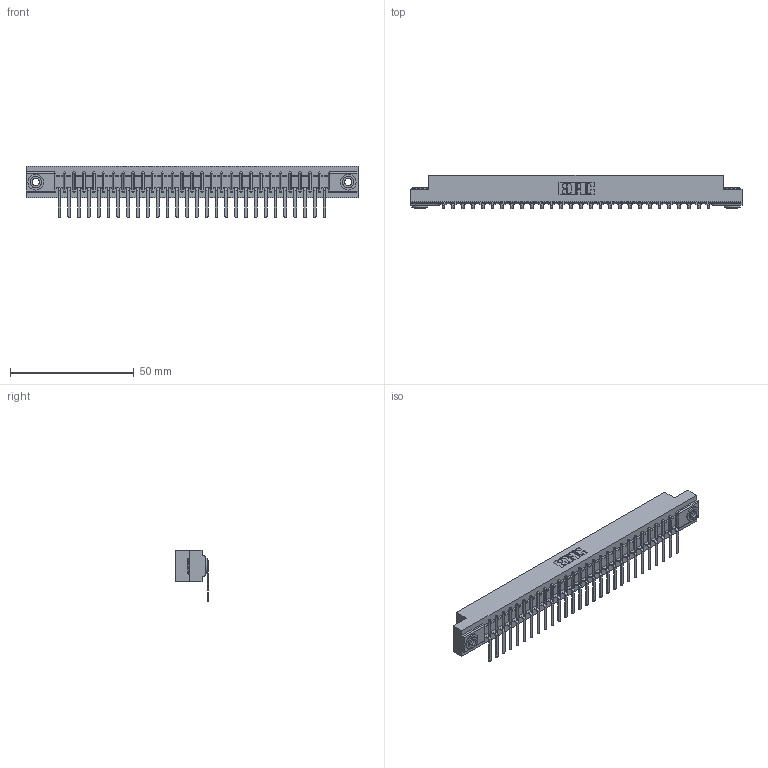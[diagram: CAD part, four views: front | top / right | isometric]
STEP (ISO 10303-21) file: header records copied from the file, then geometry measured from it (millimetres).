
FILE_DESCRIPTION (( 'STEP AP203' ), '1' );
FILE_NAME ('307-028-557-103.STEP', '2018-08-04T16:34:16', ( '' ), ( '' ), 'SwSTEP 2.0', 'SolidWorks 2016', '' );
FILE_SCHEMA (( 'CONFIG_CONTROL_DESIGN' ));
Length unit declared in the file: inch
Products named in the file (4): 307 Part_.156 Dia Mounting Holes; 307-290-002_557; 345-250-002_345-250-002-102; 307-028-557-103
Assembly tree (31 placements, depth 2):
  307-028-557-103
    307 Part_.156 Dia Mounting Holes
    307-290-002_557  x28
    345-250-002_345-250-002-102  x2
Bounding box: 133.96 x 13.36 x 20.66 mm (x, y, z)
Volume: 14307.8 mm3; surface area: 18424 mm2
Topology: 31 solids, 31 shells, 2383 faces, 7267 edges, 4762 vertices
Faces by surface type: plane 1410, cylinder 907, sphere 58, cone 8
Entity records: 27649 total; most frequent: CARTESIAN_POINT 4641, ORIENTED_EDGE 4622, DIRECTION 4531, EDGE_CURVE 2311, LINE 1755, VECTOR 1755, VERTEX_POINT 1498, AXIS2_PLACEMENT_3D 1388
